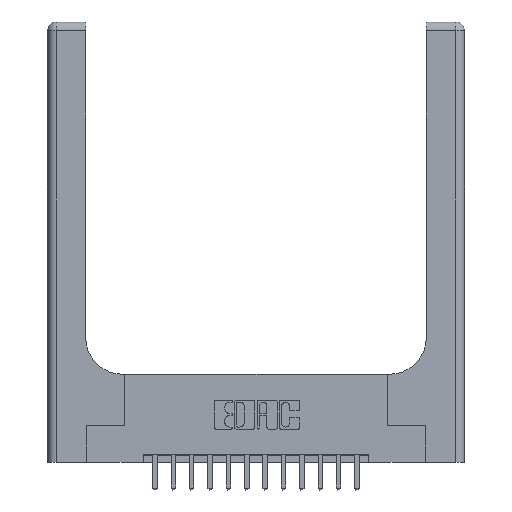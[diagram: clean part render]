
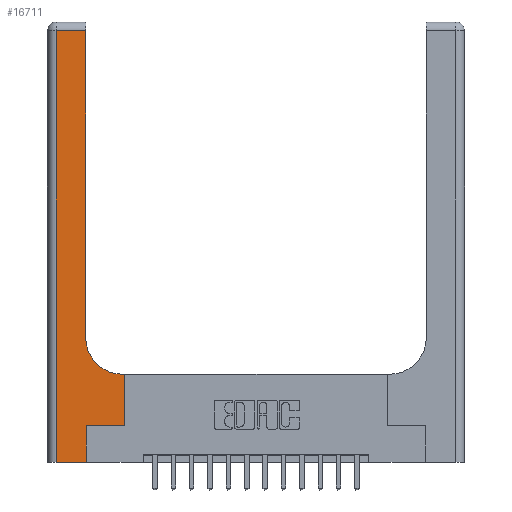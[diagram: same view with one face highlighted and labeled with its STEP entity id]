
A CAD part, top view. The second image highlights one B-rep face of the part: STEP entity #16711.
In plain terms, the highlighted planar face has unit normal (0, 0, 1).
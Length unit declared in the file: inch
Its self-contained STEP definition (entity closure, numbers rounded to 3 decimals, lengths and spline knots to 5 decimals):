
#507 = CARTESIAN_POINT ( 'NONE',  ( 0.06, 0., 0.37 ) ) ;
#1069 = VECTOR ( 'NONE', #14364, 39.37008 ) ;
#1146 = AXIS2_PLACEMENT_3D ( 'NONE', #1364, #14709, #9360 ) ;
#1364 = CARTESIAN_POINT ( 'NONE',  ( 0., 3., 0.37 ) ) ;
#2043 = CIRCLE ( 'NONE', #12311, 0.25 ) ;
#2304 = CARTESIAN_POINT ( 'NONE',  ( 0.26, 2.94, 0.37 ) ) ;
#2606 = CARTESIAN_POINT ( 'NONE',  ( 0.26, 0.85, 0.37 ) ) ;
#2874 = LINE ( 'NONE', #8963, #15951 ) ;
#3113 = CARTESIAN_POINT ( 'NONE',  ( 0.265, 0.25, 0.37 ) ) ;
#3187 = DIRECTION ( 'NONE',  ( 0., 1., 0. ) ) ;
#3198 = EDGE_LOOP ( 'NONE', ( #13016, #10615, #11916, #7464, #8175, #14828, #13789, #7597, #3963 ) ) ;
#3487 = EDGE_CURVE ( 'NONE', #8147, #12286, #16772, .T. ) ;
#3573 = CARTESIAN_POINT ( 'NONE',  ( 0.265, 0.25, 0.37 ) ) ;
#3963 = ORIENTED_EDGE ( 'NONE', *, *, #6444, .T. ) ;
#4121 = CARTESIAN_POINT ( 'NONE',  ( 0.265, 0., 0.37 ) ) ;
#4425 = CARTESIAN_POINT ( 'NONE',  ( 0.26, 3., 0.37 ) ) ;
#4880 = CARTESIAN_POINT ( 'NONE',  ( 0., 2.94, 0.37 ) ) ;
#5209 = VERTEX_POINT ( 'NONE', #3573 ) ;
#5276 = CARTESIAN_POINT ( 'NONE',  ( 0., 0., 0.37 ) ) ;
#5399 = VECTOR ( 'NONE', #14835, 39.37008 ) ;
#6074 = EDGE_CURVE ( 'NONE', #12286, #5209, #15950, .T. ) ;
#6444 = EDGE_CURVE ( 'NONE', #16848, #10361, #2043, .T. ) ;
#6722 = EDGE_CURVE ( 'NONE', #14214, #16848, #2874, .T. ) ;
#6852 = VERTEX_POINT ( 'NONE', #9582 ) ;
#7120 = LINE ( 'NONE', #16925, #1069 ) ;
#7307 = DIRECTION ( 'NONE',  ( -1., 0., 0. ) ) ;
#7464 = ORIENTED_EDGE ( 'NONE', *, *, #3487, .T. ) ;
#7597 = ORIENTED_EDGE ( 'NONE', *, *, #6722, .T. ) ;
#8147 = VERTEX_POINT ( 'NONE', #507 ) ;
#8175 = ORIENTED_EDGE ( 'NONE', *, *, #6074, .T. ) ;
#8647 = VECTOR ( 'NONE', #10716, 39.37008 ) ;
#8824 = CARTESIAN_POINT ( 'NONE',  ( 0.528, 0.6, 0.37 ) ) ;
#8855 = LINE ( 'NONE', #16076, #8647 ) ;
#8963 = CARTESIAN_POINT ( 'NONE',  ( 0.26, 0.6, 0.37 ) ) ;
#9227 = DIRECTION ( 'NONE',  ( 1., 0., 0. ) ) ;
#9360 = DIRECTION ( 'NONE',  ( -1., 0., 0. ) ) ;
#9481 = CARTESIAN_POINT ( 'NONE',  ( 0.265, 0., 0.37 ) ) ;
#9582 = CARTESIAN_POINT ( 'NONE',  ( 0.528, 0.25, 0.37 ) ) ;
#9812 = CARTESIAN_POINT ( 'NONE',  ( 0.51, 0.6, 0.37 ) ) ;
#10024 = VECTOR ( 'NONE', #7307, 39.37008 ) ;
#10206 = EDGE_CURVE ( 'NONE', #6852, #14214, #7120, .T. ) ;
#10361 = VERTEX_POINT ( 'NONE', #2606 ) ;
#10585 = EDGE_CURVE ( 'NONE', #13780, #15660, #12491, .T. ) ;
#10615 = ORIENTED_EDGE ( 'NONE', *, *, #10585, .T. ) ;
#10716 = DIRECTION ( 'NONE',  ( 0., -1., 0. ) ) ;
#11265 = VECTOR ( 'NONE', #3187, 39.37008 ) ;
#11701 = LINE ( 'NONE', #3113, #13697 ) ;
#11916 = ORIENTED_EDGE ( 'NONE', *, *, #14490, .T. ) ;
#11955 = PLANE ( 'NONE',  #1146 ) ;
#12284 = DIRECTION ( 'NONE',  ( 1., 0., 0. ) ) ;
#12286 = VERTEX_POINT ( 'NONE', #4121 ) ;
#12311 = AXIS2_PLACEMENT_3D ( 'NONE', #14964, #12416, #16298 ) ;
#12416 = DIRECTION ( 'NONE',  ( 0., 0., -1. ) ) ;
#12421 = VECTOR ( 'NONE', #9227, 39.37008 ) ;
#12441 = EDGE_CURVE ( 'NONE', #5209, #6852, #11701, .T. ) ;
#12491 = LINE ( 'NONE', #4880, #10024 ) ;
#13016 = ORIENTED_EDGE ( 'NONE', *, *, #16350, .T. ) ;
#13232 = CARTESIAN_POINT ( 'NONE',  ( 0.06, 2.94, 0.37 ) ) ;
#13697 = VECTOR ( 'NONE', #12284, 39.37008 ) ;
#13780 = VERTEX_POINT ( 'NONE', #2304 ) ;
#13789 = ORIENTED_EDGE ( 'NONE', *, *, #10206, .T. ) ;
#14214 = VERTEX_POINT ( 'NONE', #8824 ) ;
#14351 = LINE ( 'NONE', #4425, #11265 ) ;
#14364 = DIRECTION ( 'NONE',  ( 0., 1., 0. ) ) ;
#14490 = EDGE_CURVE ( 'NONE', #15660, #8147, #8855, .T. ) ;
#14553 = FACE_OUTER_BOUND ( 'NONE', #3198, .T. ) ;
#14709 = DIRECTION ( 'NONE',  ( 0., 0., -1. ) ) ;
#14828 = ORIENTED_EDGE ( 'NONE', *, *, #12441, .T. ) ;
#14835 = DIRECTION ( 'NONE',  ( 0., 1., 0. ) ) ;
#14964 = CARTESIAN_POINT ( 'NONE',  ( 0.51, 0.85, 0.37 ) ) ;
#15530 = DIRECTION ( 'NONE',  ( -1., 0., 0. ) ) ;
#15660 = VERTEX_POINT ( 'NONE', #13232 ) ;
#15950 = LINE ( 'NONE', #9481, #5399 ) ;
#15951 = VECTOR ( 'NONE', #15530, 39.37008 ) ;
#16076 = CARTESIAN_POINT ( 'NONE',  ( 0.06, 3., 0.37 ) ) ;
#16298 = DIRECTION ( 'NONE',  ( 1., 0., 0. ) ) ;
#16350 = EDGE_CURVE ( 'NONE', #10361, #13780, #14351, .T. ) ;
#16711 = ADVANCED_FACE ( 'NONE', ( #14553 ), #11955, .F. ) ;
#16772 = LINE ( 'NONE', #5276, #12421 ) ;
#16848 = VERTEX_POINT ( 'NONE', #9812 ) ;
#16925 = CARTESIAN_POINT ( 'NONE',  ( 0.528, 0.25, 0.37 ) ) ;
